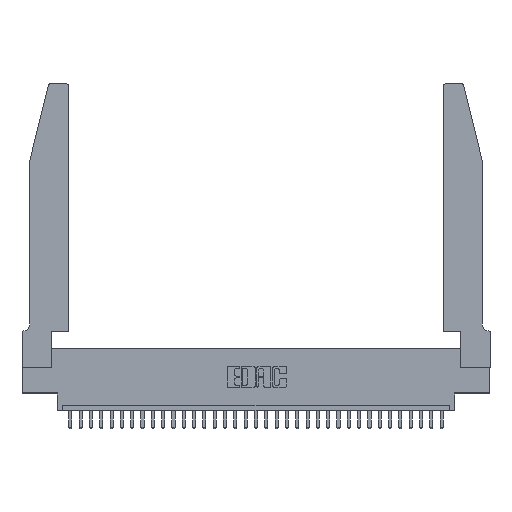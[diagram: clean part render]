
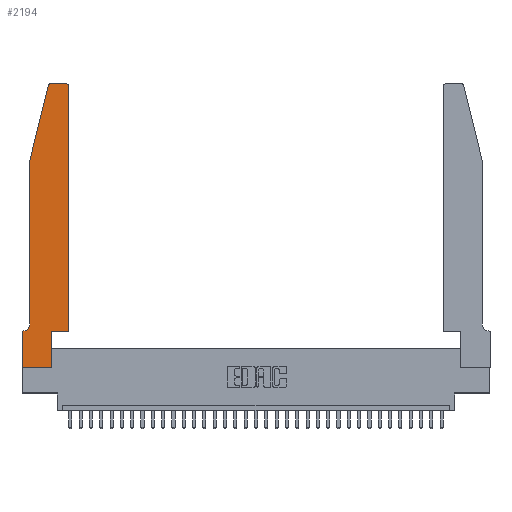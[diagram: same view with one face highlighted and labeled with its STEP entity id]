
A CAD part, top view. The second image highlights one B-rep face of the part: STEP entity #2194.
In plain terms, the highlighted planar face has unit normal (0, 0, 1).
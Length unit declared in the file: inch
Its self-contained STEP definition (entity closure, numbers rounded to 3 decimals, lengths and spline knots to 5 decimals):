
#131 = CIRCLE ( 'NONE', #21322, 0.07 ) ;
#604 = LINE ( 'NONE', #4201, #16014 ) ;
#716 = ORIENTED_EDGE ( 'NONE', *, *, #6284, .T. ) ;
#749 = CARTESIAN_POINT ( 'NONE',  ( 0.0755, 0.35, 0.37 ) ) ;
#1210 = ORIENTED_EDGE ( 'NONE', *, *, #20761, .T. ) ;
#1505 = CARTESIAN_POINT ( 'NONE',  ( 0.0755, 0.42, 0.37 ) ) ;
#1536 = FACE_OUTER_BOUND ( 'NONE', #27058, .T. ) ;
#1692 = EDGE_CURVE ( 'NONE', #18784, #11333, #2827, .T. ) ;
#1768 = VERTEX_POINT ( 'NONE', #20289 ) ;
#1897 = VERTEX_POINT ( 'NONE', #28284 ) ;
#2194 = ADVANCED_FACE ( 'NONE', ( #1536 ), #28759, .T. ) ;
#2344 = DIRECTION ( 'NONE',  ( 0., 1., 0. ) ) ;
#2635 = DIRECTION ( 'NONE',  ( 1., 0., 0. ) ) ;
#2702 = CARTESIAN_POINT ( 'NONE',  ( 0.4505, 0.35, 0.37 ) ) ;
#2827 = LINE ( 'NONE', #20174, #27907 ) ;
#2867 = CARTESIAN_POINT ( 'NONE',  ( 0.4505, 0.35, 0.37 ) ) ;
#2959 = ORIENTED_EDGE ( 'NONE', *, *, #25766, .T. ) ;
#3479 = VECTOR ( 'NONE', #8284, 39.37008 ) ;
#3854 = CARTESIAN_POINT ( 'NONE',  ( 0.2865, 0.35, 0.37 ) ) ;
#4179 = CARTESIAN_POINT ( 'NONE',  ( 0.0755, 2., 0.37 ) ) ;
#4201 = CARTESIAN_POINT ( 'NONE',  ( 0.2865, 0.35, 0.37 ) ) ;
#4214 = DIRECTION ( 'NONE',  ( 1., 0., 0. ) ) ;
#4708 = CARTESIAN_POINT ( 'NONE',  ( 0.2865, 0., 0.37 ) ) ;
#5134 = VECTOR ( 'NONE', #27136, 39.37008 ) ;
#5947 = DIRECTION ( 'NONE',  ( -0.239, -0.971, 0. ) ) ;
#6284 = EDGE_CURVE ( 'NONE', #7648, #9528, #29982, .T. ) ;
#7648 = VERTEX_POINT ( 'NONE', #2867 ) ;
#7878 = CIRCLE ( 'NONE', #11022, 0.03 ) ;
#8002 = DIRECTION ( 'NONE',  ( 1., 0., 0. ) ) ;
#8039 = DIRECTION ( 'NONE',  ( 0., 0., 1. ) ) ;
#8284 = DIRECTION ( 'NONE',  ( 1., 0., 0. ) ) ;
#9528 = VERTEX_POINT ( 'NONE', #25566 ) ;
#9803 = DIRECTION ( 'NONE',  ( -1., 0., 0. ) ) ;
#10157 = ORIENTED_EDGE ( 'NONE', *, *, #19906, .T. ) ;
#10319 = VERTEX_POINT ( 'NONE', #32471 ) ;
#10546 = CARTESIAN_POINT ( 'NONE',  ( 0., 0.35, 0.37 ) ) ;
#10755 = ORIENTED_EDGE ( 'NONE', *, *, #16070, .T. ) ;
#10879 = VECTOR ( 'NONE', #5947, 39.37008 ) ;
#11022 = AXIS2_PLACEMENT_3D ( 'NONE', #27734, #30569, #22769 ) ;
#11057 = EDGE_CURVE ( 'NONE', #10319, #14856, #17747, .T. ) ;
#11333 = VERTEX_POINT ( 'NONE', #13261 ) ;
#11789 = CARTESIAN_POINT ( 'NONE',  ( 0.284, 2.72, 0.37 ) ) ;
#11877 = ORIENTED_EDGE ( 'NONE', *, *, #31658, .T. ) ;
#12009 = DIRECTION ( 'NONE',  ( 0., 0., 1. ) ) ;
#12224 = AXIS2_PLACEMENT_3D ( 'NONE', #10546, #8039, #2635 ) ;
#12967 = DIRECTION ( 'NONE',  ( 0., -1., 0. ) ) ;
#13261 = CARTESIAN_POINT ( 'NONE',  ( 0., 0., 0.37 ) ) ;
#13719 = CIRCLE ( 'NONE', #13804, 0.03 ) ;
#13804 = AXIS2_PLACEMENT_3D ( 'NONE', #11789, #12009, #4214 ) ;
#14252 = CARTESIAN_POINT ( 'NONE',  ( 0.0755, 2., 0.37 ) ) ;
#14290 = VERTEX_POINT ( 'NONE', #1505 ) ;
#14734 = ORIENTED_EDGE ( 'NONE', *, *, #20511, .T. ) ;
#14843 = LINE ( 'NONE', #14252, #5134 ) ;
#14856 = VERTEX_POINT ( 'NONE', #4179 ) ;
#16014 = VECTOR ( 'NONE', #24816, 39.37008 ) ;
#16070 = EDGE_CURVE ( 'NONE', #14290, #22393, #131, .T. ) ;
#16324 = CARTESIAN_POINT ( 'NONE',  ( 0.0055, 0.35, 0.37 ) ) ;
#17200 = LINE ( 'NONE', #2702, #29383 ) ;
#17747 = LINE ( 'NONE', #18496, #10879 ) ;
#17795 = DIRECTION ( 'NONE',  ( 0., 0., -1. ) ) ;
#18496 = CARTESIAN_POINT ( 'NONE',  ( 0.0755, 2., 0.37 ) ) ;
#18784 = VERTEX_POINT ( 'NONE', #21020 ) ;
#19653 = VECTOR ( 'NONE', #9803, 39.37008 ) ;
#19906 = EDGE_CURVE ( 'NONE', #22393, #18784, #24588, .T. ) ;
#20174 = CARTESIAN_POINT ( 'NONE',  ( 0., 0., 0.37 ) ) ;
#20289 = CARTESIAN_POINT ( 'NONE',  ( 0.4205, 2.75, 0.37 ) ) ;
#20511 = EDGE_CURVE ( 'NONE', #11333, #22151, #26956, .T. ) ;
#20761 = EDGE_CURVE ( 'NONE', #22151, #23674, #604, .T. ) ;
#20934 = VECTOR ( 'NONE', #31991, 39.37008 ) ;
#21020 = CARTESIAN_POINT ( 'NONE',  ( 0., 0.35, 0.37 ) ) ;
#21212 = ORIENTED_EDGE ( 'NONE', *, *, #23192, .T. ) ;
#21322 = AXIS2_PLACEMENT_3D ( 'NONE', #23133, #17795, #28101 ) ;
#21414 = ORIENTED_EDGE ( 'NONE', *, *, #1692, .T. ) ;
#22148 = ORIENTED_EDGE ( 'NONE', *, *, #24430, .T. ) ;
#22151 = VERTEX_POINT ( 'NONE', #4708 ) ;
#22393 = VERTEX_POINT ( 'NONE', #16324 ) ;
#22769 = DIRECTION ( 'NONE',  ( 1., 0., 0. ) ) ;
#23133 = CARTESIAN_POINT ( 'NONE',  ( 0.0055, 0.42, 0.37 ) ) ;
#23192 = EDGE_CURVE ( 'NONE', #1897, #10319, #13719, .T. ) ;
#23602 = CARTESIAN_POINT ( 'NONE',  ( 0., 0., 0.37 ) ) ;
#23674 = VERTEX_POINT ( 'NONE', #3854 ) ;
#24430 = EDGE_CURVE ( 'NONE', #1768, #1897, #32635, .T. ) ;
#24588 = LINE ( 'NONE', #749, #20934 ) ;
#24644 = CARTESIAN_POINT ( 'NONE',  ( 0.2605, 2.75, 0.37 ) ) ;
#24816 = DIRECTION ( 'NONE',  ( 0., 1., 0. ) ) ;
#25349 = CARTESIAN_POINT ( 'NONE',  ( 0.4505, 0.35, 0.37 ) ) ;
#25566 = CARTESIAN_POINT ( 'NONE',  ( 0.4505, 2.72, 0.37 ) ) ;
#25766 = EDGE_CURVE ( 'NONE', #9528, #1768, #7878, .T. ) ;
#26956 = LINE ( 'NONE', #23602, #3479 ) ;
#27058 = EDGE_LOOP ( 'NONE', ( #22148, #21212, #31833, #30920, #10755, #10157, #21414, #14734, #1210, #11877, #716, #2959 ) ) ;
#27136 = DIRECTION ( 'NONE',  ( 0., -1., 0. ) ) ;
#27734 = CARTESIAN_POINT ( 'NONE',  ( 0.4205, 2.72, 0.37 ) ) ;
#27907 = VECTOR ( 'NONE', #12967, 39.37008 ) ;
#28101 = DIRECTION ( 'NONE',  ( -1., 0., 0. ) ) ;
#28284 = CARTESIAN_POINT ( 'NONE',  ( 0.284, 2.75, 0.37 ) ) ;
#28759 = PLANE ( 'NONE',  #12224 ) ;
#29383 = VECTOR ( 'NONE', #8002, 39.37008 ) ;
#29982 = LINE ( 'NONE', #25349, #30805 ) ;
#30569 = DIRECTION ( 'NONE',  ( 0., 0., 1. ) ) ;
#30768 = EDGE_CURVE ( 'NONE', #14856, #14290, #14843, .T. ) ;
#30805 = VECTOR ( 'NONE', #2344, 39.37008 ) ;
#30920 = ORIENTED_EDGE ( 'NONE', *, *, #30768, .T. ) ;
#31658 = EDGE_CURVE ( 'NONE', #23674, #7648, #17200, .T. ) ;
#31833 = ORIENTED_EDGE ( 'NONE', *, *, #11057, .T. ) ;
#31991 = DIRECTION ( 'NONE',  ( -1., 0., 0. ) ) ;
#32471 = CARTESIAN_POINT ( 'NONE',  ( 0.25487, 2.72718, 0.37 ) ) ;
#32635 = LINE ( 'NONE', #24644, #19653 ) ;
